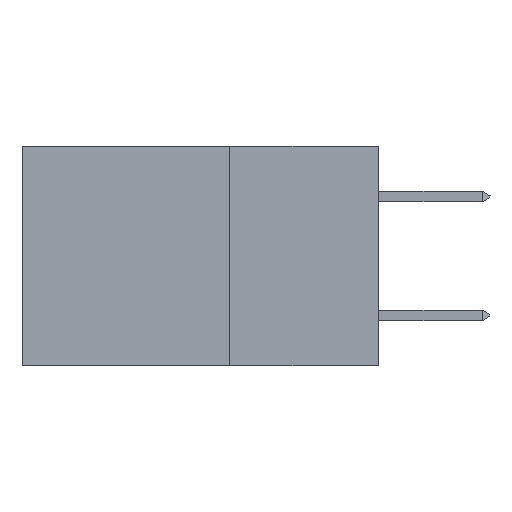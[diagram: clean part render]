
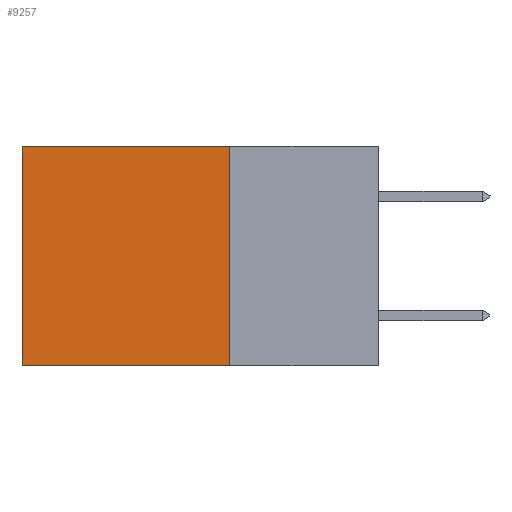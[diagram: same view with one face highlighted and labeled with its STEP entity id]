
A CAD part, left-side view. The second image highlights one B-rep face of the part: STEP entity #9257.
In plain terms, the highlighted planar face has unit normal (-1, 0, 0).
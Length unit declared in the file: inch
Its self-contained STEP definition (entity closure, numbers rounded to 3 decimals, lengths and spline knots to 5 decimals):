
#1782 = CARTESIAN_POINT ( 'NONE',  ( 0.2615, 0.6, -0.37 ) ) ;
#1788 = DIRECTION ( 'NONE',  ( 0., 0., -1. ) ) ;
#1854 = CARTESIAN_POINT ( 'NONE',  ( 0.2615, 0.25, -0.37 ) ) ;
#2018 = VERTEX_POINT ( 'NONE', #10004 ) ;
#2725 = LINE ( 'NONE', #8065, #8780 ) ;
#3428 = CARTESIAN_POINT ( 'NONE',  ( 0.2615, 0.25, -0.37 ) ) ;
#3539 = CARTESIAN_POINT ( 'NONE',  ( 0.2615, 0.6, -0.37 ) ) ;
#4346 = LINE ( 'NONE', #7805, #8587 ) ;
#4560 = DIRECTION ( 'NONE',  ( 0., 1., 0. ) ) ;
#4838 = ORIENTED_EDGE ( 'NONE', *, *, #9002, .T. ) ;
#4841 = VERTEX_POINT ( 'NONE', #11595 ) ;
#4933 = EDGE_CURVE ( 'NONE', #2018, #15257, #4346, .T. ) ;
#5705 = DIRECTION ( 'NONE',  ( 0., 1., 0. ) ) ;
#6400 = CARTESIAN_POINT ( 'NONE',  ( 0.2615, 0.25, -0.37 ) ) ;
#6625 = ORIENTED_EDGE ( 'NONE', *, *, #4933, .F. ) ;
#7805 = CARTESIAN_POINT ( 'NONE',  ( 0.2615, 0.25, -0.37 ) ) ;
#8065 = CARTESIAN_POINT ( 'NONE',  ( 0.2615, 0.25, 0. ) ) ;
#8585 = VERTEX_POINT ( 'NONE', #1782 ) ;
#8587 = VECTOR ( 'NONE', #9714, 39.37008 ) ;
#8770 = LINE ( 'NONE', #3428, #9516 ) ;
#8780 = VECTOR ( 'NONE', #5705, 39.37008 ) ;
#9002 = EDGE_CURVE ( 'NONE', #2018, #4841, #2725, .T. ) ;
#9257 = ADVANCED_FACE ( 'NONE', ( #10608 ), #14581, .F. ) ;
#9516 = VECTOR ( 'NONE', #4560, 39.37008 ) ;
#9626 = AXIS2_PLACEMENT_3D ( 'NONE', #6400, #15992, #10274 ) ;
#9714 = DIRECTION ( 'NONE',  ( 0., 0., -1. ) ) ;
#10004 = CARTESIAN_POINT ( 'NONE',  ( 0.2615, 0.25, 0. ) ) ;
#10274 = DIRECTION ( 'NONE',  ( 0., 0., -1. ) ) ;
#10608 = FACE_OUTER_BOUND ( 'NONE', #17129, .T. ) ;
#11363 = LINE ( 'NONE', #3539, #16879 ) ;
#11595 = CARTESIAN_POINT ( 'NONE',  ( 0.2615, 0.6, 0. ) ) ;
#11911 = ORIENTED_EDGE ( 'NONE', *, *, #16950, .F. ) ;
#13422 = EDGE_CURVE ( 'NONE', #4841, #8585, #11363, .T. ) ;
#14581 = PLANE ( 'NONE',  #9626 ) ;
#15257 = VERTEX_POINT ( 'NONE', #1854 ) ;
#15992 = DIRECTION ( 'NONE',  ( 1., 0., 0. ) ) ;
#16152 = ORIENTED_EDGE ( 'NONE', *, *, #13422, .T. ) ;
#16879 = VECTOR ( 'NONE', #1788, 39.37008 ) ;
#16950 = EDGE_CURVE ( 'NONE', #15257, #8585, #8770, .T. ) ;
#17129 = EDGE_LOOP ( 'NONE', ( #16152, #11911, #6625, #4838 ) ) ;
